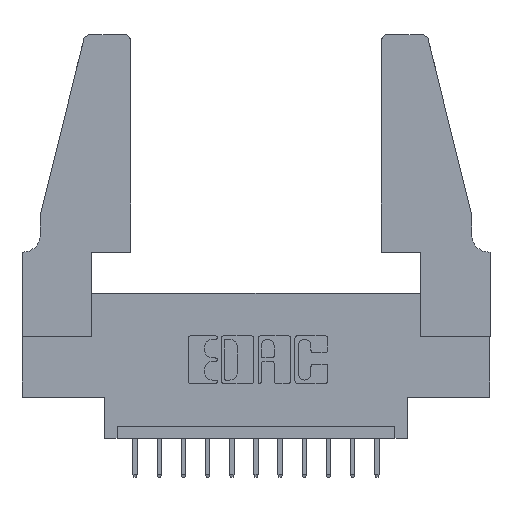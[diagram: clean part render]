
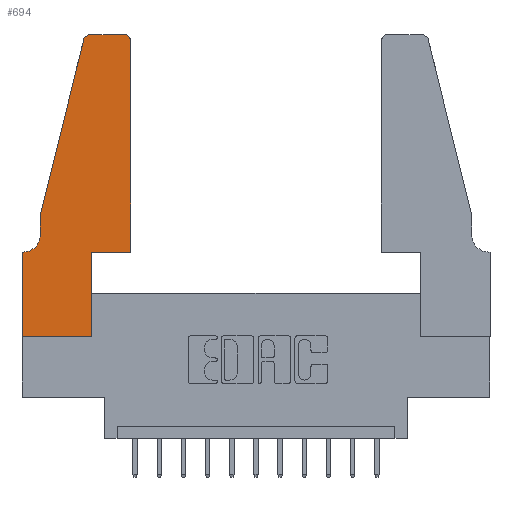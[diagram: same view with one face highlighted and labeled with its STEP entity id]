
A CAD part, top view. The second image highlights one B-rep face of the part: STEP entity #694.
In plain terms, the highlighted planar face has unit normal (0, 0, 1).
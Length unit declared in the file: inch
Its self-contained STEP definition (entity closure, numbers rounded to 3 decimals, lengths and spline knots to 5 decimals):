
#153 = CARTESIAN_POINT ( 'NONE',  ( 0.4505, 0.35, 0.37 ) ) ;
#160 = VECTOR ( 'NONE', #11649, 39.37008 ) ;
#231 = LINE ( 'NONE', #11343, #11006 ) ;
#614 = CARTESIAN_POINT ( 'NONE',  ( 0., 0.35, 0.37 ) ) ;
#626 = DIRECTION ( 'NONE',  ( 1., 0., 0. ) ) ;
#694 = ADVANCED_FACE ( 'NONE', ( #7915 ), #13645, .T. ) ;
#714 = EDGE_CURVE ( 'NONE', #8809, #13302, #8816, .T. ) ;
#741 = VECTOR ( 'NONE', #3591, 39.37008 ) ;
#884 = CARTESIAN_POINT ( 'NONE',  ( 0.2865, 0.35, 0.37 ) ) ;
#918 = VERTEX_POINT ( 'NONE', #5771 ) ;
#1061 = VERTEX_POINT ( 'NONE', #2686 ) ;
#1200 = CARTESIAN_POINT ( 'NONE',  ( 0.4205, 1.25, 0.37 ) ) ;
#1274 = DIRECTION ( 'NONE',  ( 0., -1., 0. ) ) ;
#1384 = CARTESIAN_POINT ( 'NONE',  ( 0.0055, 0.42, 0.37 ) ) ;
#1423 = VERTEX_POINT ( 'NONE', #10868 ) ;
#1890 = DIRECTION ( 'NONE',  ( 0., 0., 1. ) ) ;
#1894 = EDGE_CURVE ( 'NONE', #10802, #8809, #5305, .T. ) ;
#1934 = CARTESIAN_POINT ( 'NONE',  ( 0.4205, 1.22, 0.37 ) ) ;
#1938 = EDGE_CURVE ( 'NONE', #4110, #4612, #8188, .T. ) ;
#1971 = ORIENTED_EDGE ( 'NONE', *, *, #12050, .T. ) ;
#2170 = DIRECTION ( 'NONE',  ( 0., 0., 1. ) ) ;
#2237 = ORIENTED_EDGE ( 'NONE', *, *, #1894, .T. ) ;
#2362 = DIRECTION ( 'NONE',  ( 1., 0., 0. ) ) ;
#2499 = ORIENTED_EDGE ( 'NONE', *, *, #5513, .T. ) ;
#2588 = AXIS2_PLACEMENT_3D ( 'NONE', #1384, #9241, #3650 ) ;
#2686 = CARTESIAN_POINT ( 'NONE',  ( 0.0055, 0.35, 0.37 ) ) ;
#2718 = ORIENTED_EDGE ( 'NONE', *, *, #4377, .T. ) ;
#3106 = CIRCLE ( 'NONE', #13652, 0.03 ) ;
#3143 = EDGE_CURVE ( 'NONE', #4612, #10802, #11408, .T. ) ;
#3337 = VERTEX_POINT ( 'NONE', #1200 ) ;
#3591 = DIRECTION ( 'NONE',  ( -1., 0., 0. ) ) ;
#3650 = DIRECTION ( 'NONE',  ( -1., 0., 0. ) ) ;
#4079 = CARTESIAN_POINT ( 'NONE',  ( 0., 0., 0.37 ) ) ;
#4110 = VERTEX_POINT ( 'NONE', #614 ) ;
#4176 = VECTOR ( 'NONE', #2362, 39.37008 ) ;
#4286 = VECTOR ( 'NONE', #9284, 39.37008 ) ;
#4377 = EDGE_CURVE ( 'NONE', #918, #3337, #3106, .T. ) ;
#4567 = DIRECTION ( 'NONE',  ( 1., 0., 0. ) ) ;
#4602 = CIRCLE ( 'NONE', #9952, 0.03 ) ;
#4612 = VERTEX_POINT ( 'NONE', #4079 ) ;
#4653 = CARTESIAN_POINT ( 'NONE',  ( 0.0755, 0.5, 0.37 ) ) ;
#4674 = EDGE_LOOP ( 'NONE', ( #12612, #14640, #14182, #2499, #1971, #6280, #4678, #7028, #2237, #7644, #11493, #2718 ) ) ;
#4678 = ORIENTED_EDGE ( 'NONE', *, *, #1938, .T. ) ;
#5141 = VECTOR ( 'NONE', #1274, 39.37008 ) ;
#5305 = LINE ( 'NONE', #14788, #8353 ) ;
#5513 = EDGE_CURVE ( 'NONE', #14315, #12215, #231, .T. ) ;
#5547 = VECTOR ( 'NONE', #9474, 39.37008 ) ;
#5771 = CARTESIAN_POINT ( 'NONE',  ( 0.4505, 1.22, 0.37 ) ) ;
#5913 = EDGE_CURVE ( 'NONE', #3337, #1423, #13828, .T. ) ;
#6280 = ORIENTED_EDGE ( 'NONE', *, *, #8838, .T. ) ;
#6760 = LINE ( 'NONE', #4653, #160 ) ;
#7028 = ORIENTED_EDGE ( 'NONE', *, *, #3143, .T. ) ;
#7644 = ORIENTED_EDGE ( 'NONE', *, *, #714, .T. ) ;
#7808 = EDGE_CURVE ( 'NONE', #8402, #14315, #6760, .T. ) ;
#7915 = FACE_OUTER_BOUND ( 'NONE', #4674, .T. ) ;
#7921 = CARTESIAN_POINT ( 'NONE',  ( 0., 0., 0.37 ) ) ;
#8188 = LINE ( 'NONE', #7921, #5141 ) ;
#8219 = CARTESIAN_POINT ( 'NONE',  ( 0.2605, 1.25, 0.37 ) ) ;
#8314 = VECTOR ( 'NONE', #4567, 39.37008 ) ;
#8353 = VECTOR ( 'NONE', #11330, 39.37008 ) ;
#8402 = VERTEX_POINT ( 'NONE', #11788 ) ;
#8809 = VERTEX_POINT ( 'NONE', #884 ) ;
#8816 = LINE ( 'NONE', #13789, #4176 ) ;
#8838 = EDGE_CURVE ( 'NONE', #1061, #4110, #9492, .T. ) ;
#8935 = CARTESIAN_POINT ( 'NONE',  ( 0.0755, 0.35, 0.37 ) ) ;
#9241 = DIRECTION ( 'NONE',  ( 0., 0., -1. ) ) ;
#9284 = DIRECTION ( 'NONE',  ( -1., 0., 0. ) ) ;
#9474 = DIRECTION ( 'NONE',  ( 0., 1., 0. ) ) ;
#9492 = LINE ( 'NONE', #8935, #4286 ) ;
#9952 = AXIS2_PLACEMENT_3D ( 'NONE', #13215, #11107, #626 ) ;
#10188 = CARTESIAN_POINT ( 'NONE',  ( 0., 0., 0.37 ) ) ;
#10319 = EDGE_CURVE ( 'NONE', #1423, #8402, #4602, .T. ) ;
#10802 = VERTEX_POINT ( 'NONE', #13893 ) ;
#10868 = CARTESIAN_POINT ( 'NONE',  ( 0.284, 1.25, 0.37 ) ) ;
#11006 = VECTOR ( 'NONE', #12484, 39.37008 ) ;
#11107 = DIRECTION ( 'NONE',  ( 0., 0., 1. ) ) ;
#11330 = DIRECTION ( 'NONE',  ( 0., 1., 0. ) ) ;
#11343 = CARTESIAN_POINT ( 'NONE',  ( 0.0755, 0.5, 0.37 ) ) ;
#11403 = CARTESIAN_POINT ( 'NONE',  ( 0., 0.35, 0.37 ) ) ;
#11408 = LINE ( 'NONE', #10188, #8314 ) ;
#11493 = ORIENTED_EDGE ( 'NONE', *, *, #14005, .T. ) ;
#11550 = DIRECTION ( 'NONE',  ( 1., 0., 0. ) ) ;
#11649 = DIRECTION ( 'NONE',  ( -0.239, -0.971, 0. ) ) ;
#11712 = CARTESIAN_POINT ( 'NONE',  ( 0.4505, 0.35, 0.37 ) ) ;
#11788 = CARTESIAN_POINT ( 'NONE',  ( 0.25487, 1.22718, 0.37 ) ) ;
#11929 = CARTESIAN_POINT ( 'NONE',  ( 0.0755, 0.42, 0.37 ) ) ;
#12050 = EDGE_CURVE ( 'NONE', #12215, #1061, #13886, .T. ) ;
#12215 = VERTEX_POINT ( 'NONE', #11929 ) ;
#12416 = DIRECTION ( 'NONE',  ( 1., 0., 0. ) ) ;
#12484 = DIRECTION ( 'NONE',  ( 0., -1., 0. ) ) ;
#12488 = AXIS2_PLACEMENT_3D ( 'NONE', #11403, #2170, #11550 ) ;
#12612 = ORIENTED_EDGE ( 'NONE', *, *, #5913, .T. ) ;
#13215 = CARTESIAN_POINT ( 'NONE',  ( 0.284, 1.22, 0.37 ) ) ;
#13302 = VERTEX_POINT ( 'NONE', #153 ) ;
#13645 = PLANE ( 'NONE',  #12488 ) ;
#13652 = AXIS2_PLACEMENT_3D ( 'NONE', #1934, #1890, #12416 ) ;
#13660 = LINE ( 'NONE', #11712, #5547 ) ;
#13677 = CARTESIAN_POINT ( 'NONE',  ( 0.0755, 0.5, 0.37 ) ) ;
#13789 = CARTESIAN_POINT ( 'NONE',  ( 0.4505, 0.35, 0.37 ) ) ;
#13828 = LINE ( 'NONE', #8219, #741 ) ;
#13886 = CIRCLE ( 'NONE', #2588, 0.07 ) ;
#13893 = CARTESIAN_POINT ( 'NONE',  ( 0.2865, 0., 0.37 ) ) ;
#14005 = EDGE_CURVE ( 'NONE', #13302, #918, #13660, .T. ) ;
#14182 = ORIENTED_EDGE ( 'NONE', *, *, #7808, .T. ) ;
#14315 = VERTEX_POINT ( 'NONE', #13677 ) ;
#14640 = ORIENTED_EDGE ( 'NONE', *, *, #10319, .T. ) ;
#14788 = CARTESIAN_POINT ( 'NONE',  ( 0.2865, 0.35, 0.37 ) ) ;
